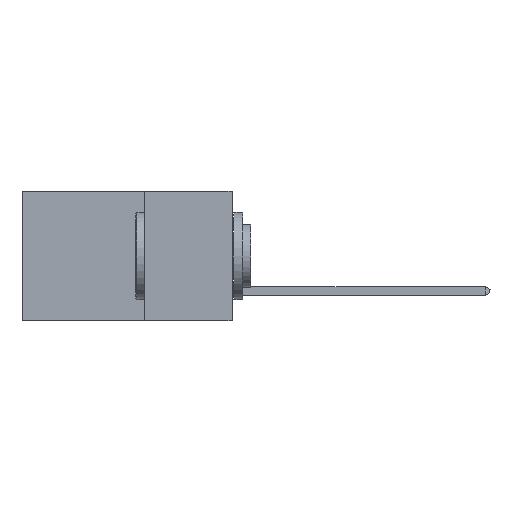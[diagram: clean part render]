
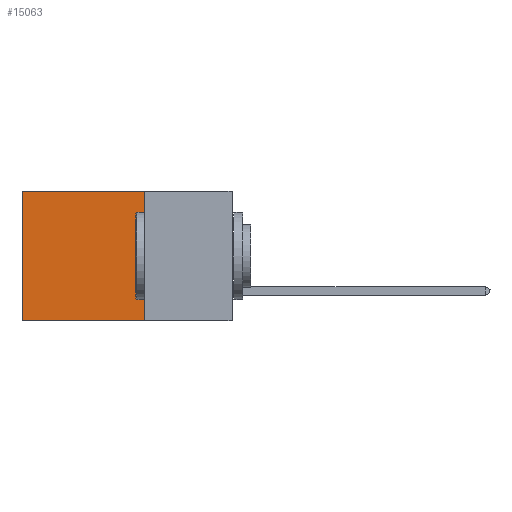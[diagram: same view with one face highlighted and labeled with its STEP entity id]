
A CAD part, left-side view. The second image highlights one B-rep face of the part: STEP entity #15063.
In plain terms, the highlighted planar face has unit normal (-1, 0, 0).
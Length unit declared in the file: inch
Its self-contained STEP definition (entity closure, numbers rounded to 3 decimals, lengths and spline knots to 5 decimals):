
#1349 = DIRECTION ( 'NONE',  ( 0., 1., 0. ) ) ;
#1380 = LINE ( 'NONE', #19575, #23036 ) ;
#1458 = LINE ( 'NONE', #19745, #16840 ) ;
#2893 = EDGE_LOOP ( 'NONE', ( #17325, #19669, #6706, #8771 ) ) ;
#3321 = EDGE_CURVE ( 'NONE', #20212, #23967, #1458, .T. ) ;
#3331 = CARTESIAN_POINT ( 'NONE',  ( 0.2875, 0.25, 0. ) ) ;
#4579 = CARTESIAN_POINT ( 'NONE',  ( 0.2875, 0.25, -0.37 ) ) ;
#6207 = DIRECTION ( 'NONE',  ( 0., 1., 0. ) ) ;
#6706 = ORIENTED_EDGE ( 'NONE', *, *, #23671, .F. ) ;
#8771 = ORIENTED_EDGE ( 'NONE', *, *, #15470, .T. ) ;
#8951 = VECTOR ( 'NONE', #1349, 39.37008 ) ;
#9879 = CARTESIAN_POINT ( 'NONE',  ( 0.2875, 0.25, 0. ) ) ;
#10719 = CARTESIAN_POINT ( 'NONE',  ( 0.2875, 0.6, 0. ) ) ;
#11931 = PLANE ( 'NONE',  #26793 ) ;
#12046 = CARTESIAN_POINT ( 'NONE',  ( 0.2875, 0.25, 0. ) ) ;
#13117 = EDGE_CURVE ( 'NONE', #24602, #23967, #1380, .T. ) ;
#14767 = LINE ( 'NONE', #3331, #20326 ) ;
#15063 = ADVANCED_FACE ( 'NONE', ( #26773 ), #11931, .F. ) ;
#15470 = EDGE_CURVE ( 'NONE', #24113, #20212, #28853, .T. ) ;
#16423 = DIRECTION ( 'NONE',  ( 0., 0., -1. ) ) ;
#16840 = VECTOR ( 'NONE', #28836, 39.37008 ) ;
#17325 = ORIENTED_EDGE ( 'NONE', *, *, #3321, .T. ) ;
#19000 = DIRECTION ( 'NONE',  ( 0., 0., -1. ) ) ;
#19575 = CARTESIAN_POINT ( 'NONE',  ( 0.2875, 0.25, -0.37 ) ) ;
#19669 = ORIENTED_EDGE ( 'NONE', *, *, #13117, .F. ) ;
#19745 = CARTESIAN_POINT ( 'NONE',  ( 0.2875, 0.6, 0. ) ) ;
#20019 = CARTESIAN_POINT ( 'NONE',  ( 0.2875, 0.25, 0. ) ) ;
#20212 = VERTEX_POINT ( 'NONE', #10719 ) ;
#20326 = VECTOR ( 'NONE', #19000, 39.37008 ) ;
#23036 = VECTOR ( 'NONE', #6207, 39.37008 ) ;
#23671 = EDGE_CURVE ( 'NONE', #24113, #24602, #14767, .T. ) ;
#23967 = VERTEX_POINT ( 'NONE', #23970 ) ;
#23970 = CARTESIAN_POINT ( 'NONE',  ( 0.2875, 0.6, -0.37 ) ) ;
#24113 = VERTEX_POINT ( 'NONE', #20019 ) ;
#24602 = VERTEX_POINT ( 'NONE', #4579 ) ;
#25595 = DIRECTION ( 'NONE',  ( 1., 0., 0. ) ) ;
#26773 = FACE_OUTER_BOUND ( 'NONE', #2893, .T. ) ;
#26793 = AXIS2_PLACEMENT_3D ( 'NONE', #12046, #25595, #16423 ) ;
#28836 = DIRECTION ( 'NONE',  ( 0., 0., -1. ) ) ;
#28853 = LINE ( 'NONE', #9879, #8951 ) ;
